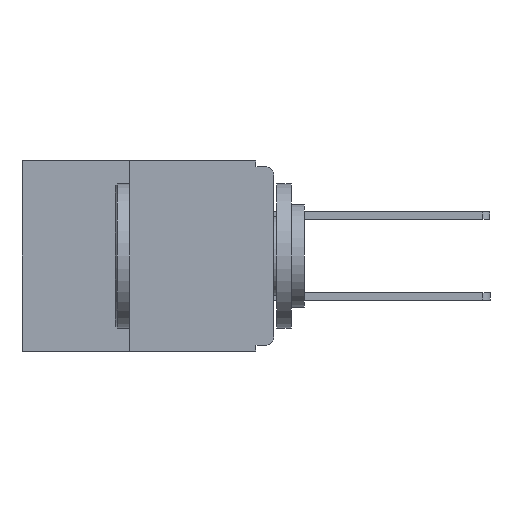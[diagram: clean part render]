
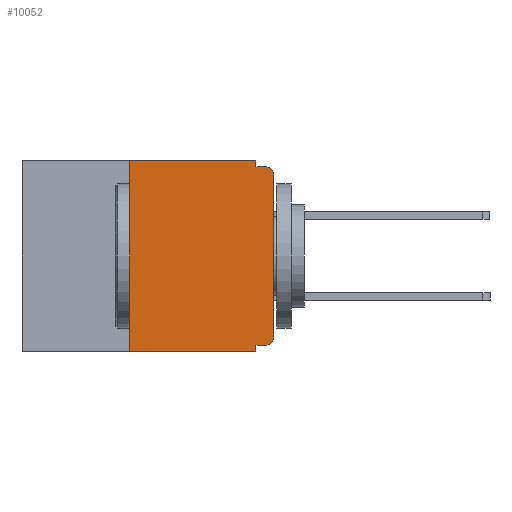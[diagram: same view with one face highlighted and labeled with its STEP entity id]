
A CAD part, left-side view. The second image highlights one B-rep face of the part: STEP entity #10052.
In plain terms, the highlighted planar face has unit normal (-1, 0, 0).
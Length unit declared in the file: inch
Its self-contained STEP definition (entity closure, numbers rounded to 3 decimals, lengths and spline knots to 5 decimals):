
#6 = VECTOR ( 'NONE', #3163, 39.37008 ) ;
#354 = CARTESIAN_POINT ( 'NONE',  ( 0., 0.031, -0.33 ) ) ;
#453 = ORIENTED_EDGE ( 'NONE', *, *, #13564, .F. ) ;
#521 = VERTEX_POINT ( 'NONE', #11519 ) ;
#942 = PLANE ( 'NONE',  #1025 ) ;
#1025 = AXIS2_PLACEMENT_3D ( 'NONE', #15769, #10580, #2287 ) ;
#1037 = CARTESIAN_POINT ( 'NONE',  ( 0., 0.25, 0. ) ) ;
#1426 = ORIENTED_EDGE ( 'NONE', *, *, #2725, .T. ) ;
#1441 = EDGE_CURVE ( 'NONE', #2355, #3212, #14045, .T. ) ;
#1586 = AXIS2_PLACEMENT_3D ( 'NONE', #1914, #11553, #3302 ) ;
#1914 = CARTESIAN_POINT ( 'NONE',  ( 0., 0.015, -0.025 ) ) ;
#1996 = VECTOR ( 'NONE', #11401, 39.37008 ) ;
#2008 = CARTESIAN_POINT ( 'NONE',  ( 0., 0.031, 0. ) ) ;
#2058 = ORIENTED_EDGE ( 'NONE', *, *, #16494, .F. ) ;
#2254 = VECTOR ( 'NONE', #12616, 39.37008 ) ;
#2275 = FACE_OUTER_BOUND ( 'NONE', #14504, .T. ) ;
#2287 = DIRECTION ( 'NONE',  ( 0., 0., -1. ) ) ;
#2355 = VERTEX_POINT ( 'NONE', #1037 ) ;
#2635 = AXIS2_PLACEMENT_3D ( 'NONE', #7180, #8842, #11675 ) ;
#2725 = EDGE_CURVE ( 'NONE', #15366, #13925, #15254, .T. ) ;
#2786 = VERTEX_POINT ( 'NONE', #16917 ) ;
#3033 = CARTESIAN_POINT ( 'NONE',  ( 0., 0.25, -0.33 ) ) ;
#3034 = VECTOR ( 'NONE', #11947, 39.37008 ) ;
#3163 = DIRECTION ( 'NONE',  ( 0., -1., 0. ) ) ;
#3212 = VERTEX_POINT ( 'NONE', #2008 ) ;
#3302 = DIRECTION ( 'NONE',  ( 0., 0., -1. ) ) ;
#3699 = LINE ( 'NONE', #6013, #6 ) ;
#3714 = CARTESIAN_POINT ( 'NONE',  ( 0., 0., -0.01 ) ) ;
#4231 = LINE ( 'NONE', #5723, #7146 ) ;
#5145 = CARTESIAN_POINT ( 'NONE',  ( 0., 0.031, -0.32 ) ) ;
#5235 = DIRECTION ( 'NONE',  ( 0., 0., 1. ) ) ;
#5723 = CARTESIAN_POINT ( 'NONE',  ( 0., 0., -0.32 ) ) ;
#5869 = CARTESIAN_POINT ( 'NONE',  ( 0., 0., -0.305 ) ) ;
#6013 = CARTESIAN_POINT ( 'NONE',  ( 0., 0.437, -0.33 ) ) ;
#6081 = VERTEX_POINT ( 'NONE', #10165 ) ;
#6218 = ORIENTED_EDGE ( 'NONE', *, *, #11581, .F. ) ;
#7146 = VECTOR ( 'NONE', #16326, 39.37008 ) ;
#7180 = CARTESIAN_POINT ( 'NONE',  ( 0., 0.015, -0.305 ) ) ;
#7321 = ORIENTED_EDGE ( 'NONE', *, *, #1441, .F. ) ;
#7446 = CARTESIAN_POINT ( 'NONE',  ( 0., 0., -0.025 ) ) ;
#7745 = CARTESIAN_POINT ( 'NONE',  ( 0., 0.031, 0. ) ) ;
#8842 = DIRECTION ( 'NONE',  ( -1., 0., 0. ) ) ;
#9182 = ORIENTED_EDGE ( 'NONE', *, *, #16783, .F. ) ;
#9244 = LINE ( 'NONE', #3033, #2254 ) ;
#9510 = DIRECTION ( 'NONE',  ( 0., -1., 0. ) ) ;
#9656 = VECTOR ( 'NONE', #10446, 39.37008 ) ;
#9784 = VERTEX_POINT ( 'NONE', #5145 ) ;
#10052 = ADVANCED_FACE ( 'NONE', ( #2275 ), #942, .F. ) ;
#10165 = CARTESIAN_POINT ( 'NONE',  ( 0., 0.031, -0.33 ) ) ;
#10272 = VECTOR ( 'NONE', #5235, 39.37008 ) ;
#10392 = EDGE_CURVE ( 'NONE', #10968, #2786, #10923, .T. ) ;
#10446 = DIRECTION ( 'NONE',  ( 0., 0., -1. ) ) ;
#10580 = DIRECTION ( 'NONE',  ( 1., 0., 0. ) ) ;
#10598 = VECTOR ( 'NONE', #9510, 39.37008 ) ;
#10628 = EDGE_CURVE ( 'NONE', #13925, #10968, #14133, .T. ) ;
#10822 = LINE ( 'NONE', #3714, #3034 ) ;
#10923 = CIRCLE ( 'NONE', #1586, 0.015 ) ;
#10968 = VERTEX_POINT ( 'NONE', #7446 ) ;
#11276 = CARTESIAN_POINT ( 'NONE',  ( 0., 0.25, -0.33 ) ) ;
#11401 = DIRECTION ( 'NONE',  ( 0., 0., -1. ) ) ;
#11475 = ORIENTED_EDGE ( 'NONE', *, *, #10392, .T. ) ;
#11519 = CARTESIAN_POINT ( 'NONE',  ( 0., 0.031, -0.01 ) ) ;
#11553 = DIRECTION ( 'NONE',  ( -1., 0., 0. ) ) ;
#11581 = EDGE_CURVE ( 'NONE', #9784, #6081, #16359, .T. ) ;
#11675 = DIRECTION ( 'NONE',  ( 0., 0., -1. ) ) ;
#11947 = DIRECTION ( 'NONE',  ( 0., -1., 0. ) ) ;
#11950 = CARTESIAN_POINT ( 'NONE',  ( 0., 0.015, -0.32 ) ) ;
#12152 = VERTEX_POINT ( 'NONE', #11276 ) ;
#12161 = CARTESIAN_POINT ( 'NONE',  ( 0., 0.437, 0. ) ) ;
#12616 = DIRECTION ( 'NONE',  ( 0., 0., 1. ) ) ;
#13313 = EDGE_CURVE ( 'NONE', #12152, #6081, #3699, .T. ) ;
#13518 = LINE ( 'NONE', #7745, #9656 ) ;
#13564 = EDGE_CURVE ( 'NONE', #521, #2786, #10822, .T. ) ;
#13891 = ORIENTED_EDGE ( 'NONE', *, *, #15936, .F. ) ;
#13925 = VERTEX_POINT ( 'NONE', #5869 ) ;
#14045 = LINE ( 'NONE', #12161, #10598 ) ;
#14106 = ORIENTED_EDGE ( 'NONE', *, *, #10628, .T. ) ;
#14133 = LINE ( 'NONE', #14599, #10272 ) ;
#14504 = EDGE_LOOP ( 'NONE', ( #14106, #11475, #453, #9182, #7321, #13891, #15487, #6218, #2058, #1426 ) ) ;
#14599 = CARTESIAN_POINT ( 'NONE',  ( 0., 0., 0. ) ) ;
#15254 = CIRCLE ( 'NONE', #2635, 0.015 ) ;
#15366 = VERTEX_POINT ( 'NONE', #11950 ) ;
#15487 = ORIENTED_EDGE ( 'NONE', *, *, #13313, .T. ) ;
#15769 = CARTESIAN_POINT ( 'NONE',  ( 0., 0.437, 0. ) ) ;
#15936 = EDGE_CURVE ( 'NONE', #12152, #2355, #9244, .T. ) ;
#16326 = DIRECTION ( 'NONE',  ( 0., 1., 0. ) ) ;
#16359 = LINE ( 'NONE', #354, #1996 ) ;
#16494 = EDGE_CURVE ( 'NONE', #15366, #9784, #4231, .T. ) ;
#16783 = EDGE_CURVE ( 'NONE', #3212, #521, #13518, .T. ) ;
#16917 = CARTESIAN_POINT ( 'NONE',  ( 0., 0.015, -0.01 ) ) ;
